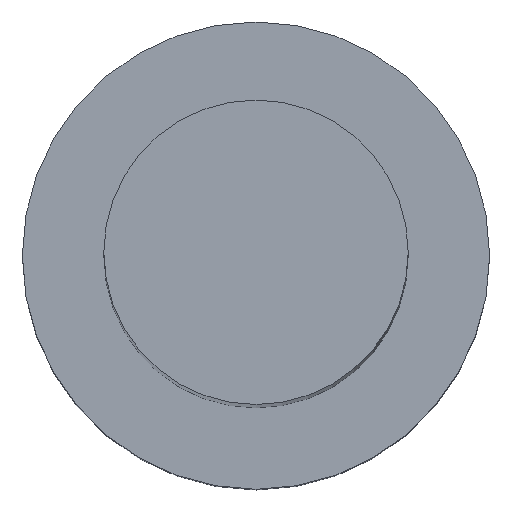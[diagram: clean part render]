
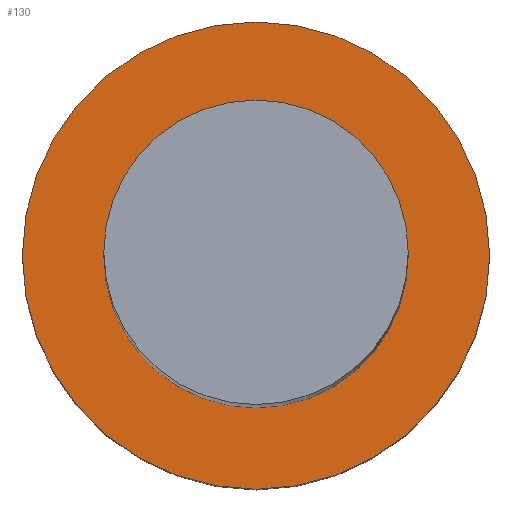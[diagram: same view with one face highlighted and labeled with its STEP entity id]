
A CAD part, top view. The second image highlights one B-rep face of the part: STEP entity #130.
In plain terms, the highlighted planar face has unit normal (0, 0, 1).
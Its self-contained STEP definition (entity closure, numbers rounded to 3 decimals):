
#7 = ORIENTED_EDGE ( 'NONE', *, *, #219, .T. ) ;
#12 = DIRECTION ( 'NONE',  ( 1., 0., 0. ) ) ;
#18 = CARTESIAN_POINT ( 'NONE',  ( -2.54, 0., -37.338 ) ) ;
#23 = DIRECTION ( 'NONE',  ( 1., 0., 0. ) ) ;
#38 = DIRECTION ( 'NONE',  ( 1., 0., 0. ) ) ;
#45 = EDGE_CURVE ( 'NONE', #119, #183, #248, .T. ) ;
#47 = CARTESIAN_POINT ( 'NONE',  ( 0., 0., -37.338 ) ) ;
#51 = FACE_BOUND ( 'NONE', #191, .T. ) ;
#69 = DIRECTION ( 'NONE',  ( 1., 0., 0. ) ) ;
#70 = AXIS2_PLACEMENT_3D ( 'NONE', #221, #170, #38 ) ;
#75 = EDGE_CURVE ( 'NONE', #232, #257, #120, .T. ) ;
#83 = ORIENTED_EDGE ( 'NONE', *, *, #45, .T. ) ;
#97 = AXIS2_PLACEMENT_3D ( 'NONE', #292, #156, #23 ) ;
#101 = CARTESIAN_POINT ( 'NONE',  ( 0., 0., -37.338 ) ) ;
#105 = CARTESIAN_POINT ( 'NONE',  ( 2.54, 0., -37.338 ) ) ;
#119 = VERTEX_POINT ( 'NONE', #105 ) ;
#120 = CIRCLE ( 'NONE', #213, 3.899 ) ;
#124 = CARTESIAN_POINT ( 'NONE',  ( 0., 0., -37.338 ) ) ;
#125 = ORIENTED_EDGE ( 'NONE', *, *, #281, .T. ) ;
#126 = DIRECTION ( 'NONE',  ( 1., 0., 0. ) ) ;
#130 = ADVANCED_FACE ( 'NONE', ( #242, #51 ), #246, .T. ) ;
#134 = CARTESIAN_POINT ( 'NONE',  ( 0., 3.899, -37.338 ) ) ;
#147 = CIRCLE ( 'NONE', #240, 2.54 ) ;
#148 = DIRECTION ( 'NONE',  ( 0., 0., -1. ) ) ;
#155 = CIRCLE ( 'NONE', #97, 3.899 ) ;
#156 = DIRECTION ( 'NONE',  ( 0., 0., 1. ) ) ;
#170 = DIRECTION ( 'NONE',  ( 0., 0., 1. ) ) ;
#179 = AXIS2_PLACEMENT_3D ( 'NONE', #124, #148, #12 ) ;
#183 = VERTEX_POINT ( 'NONE', #18 ) ;
#191 = EDGE_LOOP ( 'NONE', ( #83, #125 ) ) ;
#208 = DIRECTION ( 'NONE',  ( 0., 0., -1. ) ) ;
#213 = AXIS2_PLACEMENT_3D ( 'NONE', #101, #264, #126 ) ;
#219 = EDGE_CURVE ( 'NONE', #257, #232, #155, .T. ) ;
#221 = CARTESIAN_POINT ( 'NONE',  ( 0., 0., -37.338 ) ) ;
#229 = CARTESIAN_POINT ( 'NONE',  ( 0., -3.899, -37.338 ) ) ;
#231 = ORIENTED_EDGE ( 'NONE', *, *, #75, .T. ) ;
#232 = VERTEX_POINT ( 'NONE', #134 ) ;
#240 = AXIS2_PLACEMENT_3D ( 'NONE', #47, #208, #69 ) ;
#242 = FACE_OUTER_BOUND ( 'NONE', #260, .T. ) ;
#246 = PLANE ( 'NONE',  #70 ) ;
#248 = CIRCLE ( 'NONE', #179, 2.54 ) ;
#257 = VERTEX_POINT ( 'NONE', #229 ) ;
#260 = EDGE_LOOP ( 'NONE', ( #231, #7 ) ) ;
#264 = DIRECTION ( 'NONE',  ( 0., 0., 1. ) ) ;
#281 = EDGE_CURVE ( 'NONE', #183, #119, #147, .T. ) ;
#292 = CARTESIAN_POINT ( 'NONE',  ( 0., 0., -37.338 ) ) ;
